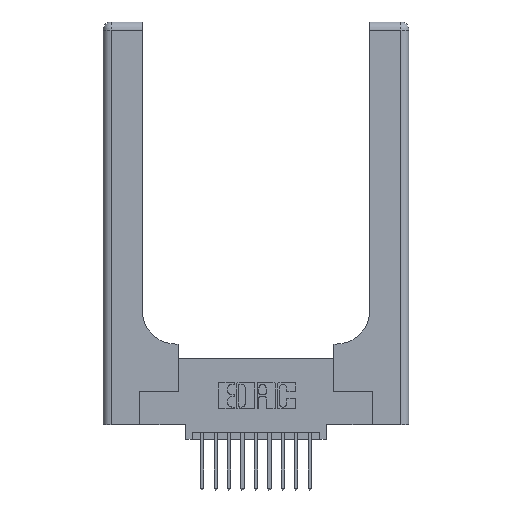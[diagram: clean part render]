
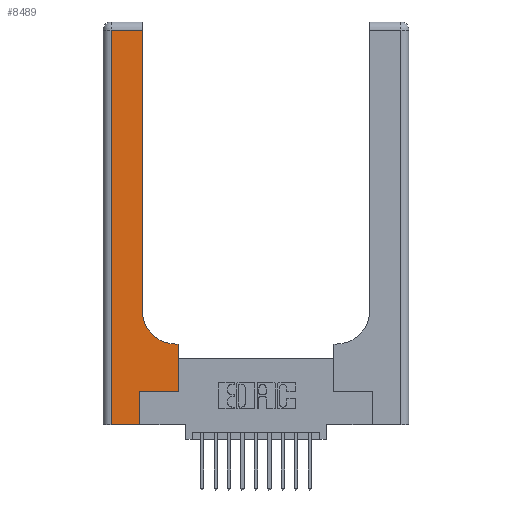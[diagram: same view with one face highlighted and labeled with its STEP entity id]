
A CAD part, top view. The second image highlights one B-rep face of the part: STEP entity #8489.
In plain terms, the highlighted planar face has unit normal (0, 0, 1).
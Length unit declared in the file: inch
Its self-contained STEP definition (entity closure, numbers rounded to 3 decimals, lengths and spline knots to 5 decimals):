
#582 = DIRECTION ( 'NONE',  ( 1., 0., 0. ) ) ;
#1641 = LINE ( 'NONE', #14358, #15413 ) ;
#2373 = ORIENTED_EDGE ( 'NONE', *, *, #8858, .T. ) ;
#2428 = LINE ( 'NONE', #15625, #15741 ) ;
#2689 = DIRECTION ( 'NONE',  ( -1., 0., 0. ) ) ;
#2701 = VERTEX_POINT ( 'NONE', #16390 ) ;
#2722 = CARTESIAN_POINT ( 'NONE',  ( 0.2915, 3., 0.37 ) ) ;
#2967 = ORIENTED_EDGE ( 'NONE', *, *, #4325, .T. ) ;
#3077 = EDGE_CURVE ( 'NONE', #10565, #10368, #9530, .T. ) ;
#3080 = EDGE_CURVE ( 'NONE', #9990, #2701, #2428, .T. ) ;
#3313 = DIRECTION ( 'NONE',  ( 0., 1., 0. ) ) ;
#3450 = ORIENTED_EDGE ( 'NONE', *, *, #12238, .T. ) ;
#3555 = CARTESIAN_POINT ( 'NONE',  ( 0.2915, 0.85, 0.37 ) ) ;
#3588 = DIRECTION ( 'NONE',  ( 0., -1., 0. ) ) ;
#3754 = DIRECTION ( 'NONE',  ( -1., 0., 0. ) ) ;
#4107 = DIRECTION ( 'NONE',  ( 0., 1., 0. ) ) ;
#4169 = VERTEX_POINT ( 'NONE', #6059 ) ;
#4262 = CARTESIAN_POINT ( 'NONE',  ( 0.5585, 0.25, 0.37 ) ) ;
#4295 = VECTOR ( 'NONE', #13675, 39.37008 ) ;
#4324 = LINE ( 'NONE', #2722, #14185 ) ;
#4325 = EDGE_CURVE ( 'NONE', #4169, #16448, #10512, .T. ) ;
#4379 = AXIS2_PLACEMENT_3D ( 'NONE', #15555, #15551, #15504 ) ;
#4626 = VECTOR ( 'NONE', #582, 39.37008 ) ;
#4782 = EDGE_CURVE ( 'NONE', #2701, #13830, #10883, .T. ) ;
#5094 = ORIENTED_EDGE ( 'NONE', *, *, #3077, .T. ) ;
#5458 = CARTESIAN_POINT ( 'NONE',  ( 0.269, 0., 0.37 ) ) ;
#5877 = DIRECTION ( 'NONE',  ( 0., 0., -1. ) ) ;
#6034 = CARTESIAN_POINT ( 'NONE',  ( 0.269, 0.25, 0.37 ) ) ;
#6059 = CARTESIAN_POINT ( 'NONE',  ( 0.2915, 2.94, 0.37 ) ) ;
#6256 = CARTESIAN_POINT ( 'NONE',  ( 0.06, 3., 0.37 ) ) ;
#6675 = CARTESIAN_POINT ( 'NONE',  ( 0.5415, 0.6, 0.37 ) ) ;
#7081 = CARTESIAN_POINT ( 'NONE',  ( 0.5585, 0.6, 0.37 ) ) ;
#7412 = VECTOR ( 'NONE', #3754, 39.37008 ) ;
#7619 = CARTESIAN_POINT ( 'NONE',  ( 0.06, 2.94, 0.37 ) ) ;
#7666 = AXIS2_PLACEMENT_3D ( 'NONE', #9792, #5877, #14766 ) ;
#7860 = ORIENTED_EDGE ( 'NONE', *, *, #3080, .T. ) ;
#8156 = LINE ( 'NONE', #14879, #4626 ) ;
#8489 = ADVANCED_FACE ( 'NONE', ( #13802 ), #13537, .F. ) ;
#8858 = EDGE_CURVE ( 'NONE', #10368, #4169, #4324, .T. ) ;
#9530 = CIRCLE ( 'NONE', #4379, 0.25 ) ;
#9792 = CARTESIAN_POINT ( 'NONE',  ( 0., 3., 0.37 ) ) ;
#9878 = VERTEX_POINT ( 'NONE', #14196 ) ;
#9990 = VERTEX_POINT ( 'NONE', #5458 ) ;
#10368 = VERTEX_POINT ( 'NONE', #3555 ) ;
#10512 = LINE ( 'NONE', #11622, #7412 ) ;
#10565 = VERTEX_POINT ( 'NONE', #6675 ) ;
#10883 = LINE ( 'NONE', #6034, #4295 ) ;
#11622 = CARTESIAN_POINT ( 'NONE',  ( 0., 2.94, 0.37 ) ) ;
#11825 = VERTEX_POINT ( 'NONE', #7081 ) ;
#12238 = EDGE_CURVE ( 'NONE', #9878, #9990, #8156, .T. ) ;
#12449 = EDGE_CURVE ( 'NONE', #11825, #10565, #1641, .T. ) ;
#12867 = ORIENTED_EDGE ( 'NONE', *, *, #12449, .T. ) ;
#12879 = VECTOR ( 'NONE', #3313, 39.37008 ) ;
#13537 = PLANE ( 'NONE',  #7666 ) ;
#13675 = DIRECTION ( 'NONE',  ( 1., 0., 0. ) ) ;
#13802 = FACE_OUTER_BOUND ( 'NONE', #16053, .T. ) ;
#13830 = VERTEX_POINT ( 'NONE', #4262 ) ;
#14185 = VECTOR ( 'NONE', #4107, 39.37008 ) ;
#14196 = CARTESIAN_POINT ( 'NONE',  ( 0.06, 0., 0.37 ) ) ;
#14207 = VECTOR ( 'NONE', #3588, 39.37008 ) ;
#14223 = ORIENTED_EDGE ( 'NONE', *, *, #15380, .T. ) ;
#14358 = CARTESIAN_POINT ( 'NONE',  ( 0.2915, 0.6, 0.37 ) ) ;
#14535 = ORIENTED_EDGE ( 'NONE', *, *, #4782, .T. ) ;
#14582 = LINE ( 'NONE', #6256, #14207 ) ;
#14766 = DIRECTION ( 'NONE',  ( -1., 0., 0. ) ) ;
#14879 = CARTESIAN_POINT ( 'NONE',  ( 0., 0., 0.37 ) ) ;
#14915 = CARTESIAN_POINT ( 'NONE',  ( 0.5585, 0.25, 0.37 ) ) ;
#15380 = EDGE_CURVE ( 'NONE', #13830, #11825, #16568, .T. ) ;
#15413 = VECTOR ( 'NONE', #2689, 39.37008 ) ;
#15504 = DIRECTION ( 'NONE',  ( 1., 0., 0. ) ) ;
#15551 = DIRECTION ( 'NONE',  ( 0., 0., -1. ) ) ;
#15555 = CARTESIAN_POINT ( 'NONE',  ( 0.5415, 0.85, 0.37 ) ) ;
#15609 = DIRECTION ( 'NONE',  ( 0., 1., 0. ) ) ;
#15625 = CARTESIAN_POINT ( 'NONE',  ( 0.269, 0., 0.37 ) ) ;
#15648 = ORIENTED_EDGE ( 'NONE', *, *, #16432, .T. ) ;
#15741 = VECTOR ( 'NONE', #15609, 39.37008 ) ;
#16053 = EDGE_LOOP ( 'NONE', ( #2373, #2967, #15648, #3450, #7860, #14535, #14223, #12867, #5094 ) ) ;
#16390 = CARTESIAN_POINT ( 'NONE',  ( 0.269, 0.25, 0.37 ) ) ;
#16432 = EDGE_CURVE ( 'NONE', #16448, #9878, #14582, .T. ) ;
#16448 = VERTEX_POINT ( 'NONE', #7619 ) ;
#16568 = LINE ( 'NONE', #14915, #12879 ) ;
